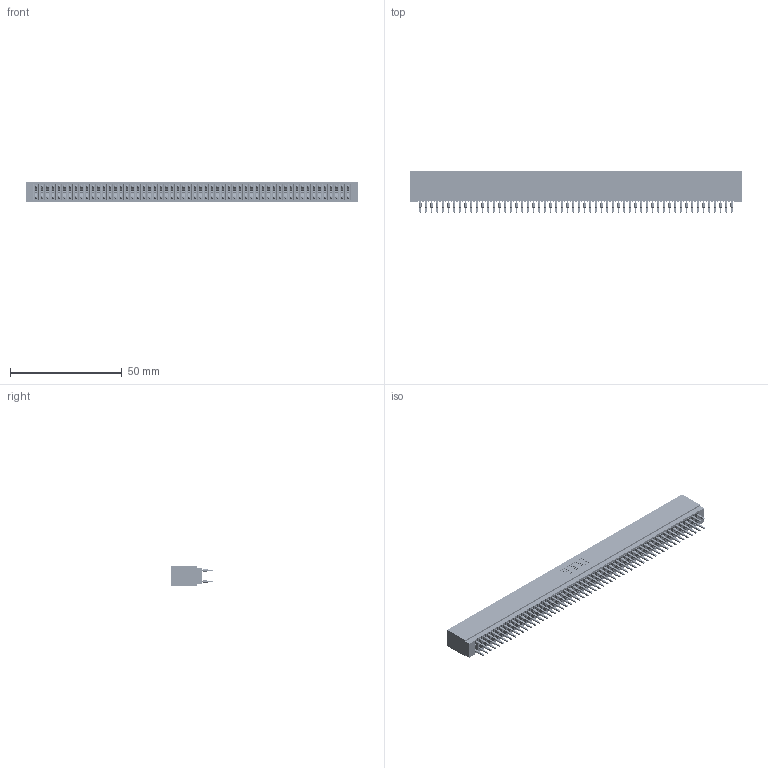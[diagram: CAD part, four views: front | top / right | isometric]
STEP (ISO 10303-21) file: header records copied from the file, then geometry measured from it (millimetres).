
FILE_DESCRIPTION (( 'STEP AP203' ), '1' );
FILE_NAME ('725-112-520-201.STEP', '2026-02-24T20:33:14', ( '' ), ( '' ), 'SwSTEP 2.0', 'SolidWorks 2023', '' );
FILE_SCHEMA (( 'CONFIG_CONTROL_DESIGN' ));
Length unit declared in the file: millimetre
Products named in the file (3): 745-292-001_520; 725-112-520-201; 725 Part_Insulator Option - 01
Assembly tree (113 placements, depth 2):
  725-112-520-201
    725 Part_Insulator Option - 01
    745-292-001_520  x112
Bounding box: 148.84 x 18.8 x 8.89 mm (x, y, z)
Volume: 11613.7 mm3; surface area: 24187.3 mm2
Topology: 113 solids, 113 shells, 10119 faces, 27190 edges, 17080 vertices
Faces by surface type: plane 5207, bspline 2240, cylinder 2000, torus 672
Entity records: 92330 total; most frequent: CARTESIAN_POINT 16511, ORIENTED_EDGE 15974, DIRECTION 13945, EDGE_CURVE 7987, LINE 7469, VECTOR 7469, VERTEX_POINT 5092, AXIS2_PLACEMENT_3D 3238
